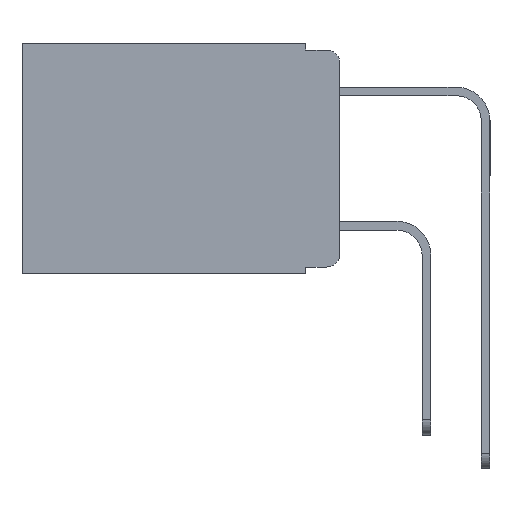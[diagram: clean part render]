
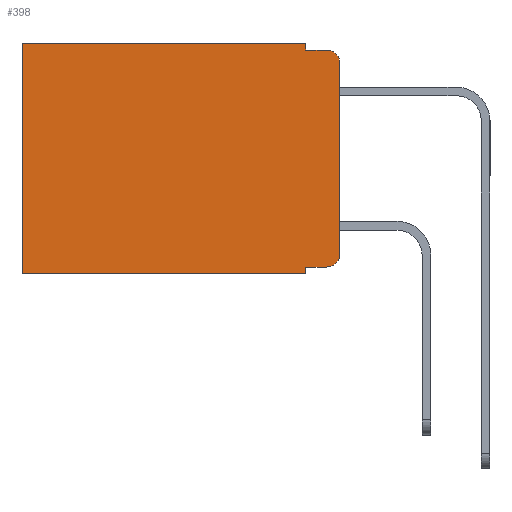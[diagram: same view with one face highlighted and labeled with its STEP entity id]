
A CAD part, left-side view. The second image highlights one B-rep face of the part: STEP entity #398.
In plain terms, the highlighted planar face has unit normal (-1, 0, 0).
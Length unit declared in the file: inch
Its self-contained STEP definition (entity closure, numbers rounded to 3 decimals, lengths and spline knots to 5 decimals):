
#398 = ADVANCED_FACE ( 'NONE', ( #4030 ), #1964, .F. ) ;
#579 = DIRECTION ( 'NONE',  ( 0., 0., -1. ) ) ;
#777 = CARTESIAN_POINT ( 'NONE',  ( 0.298, 0.02, -0.01 ) ) ;
#1148 = ORIENTED_EDGE ( 'NONE', *, *, #8814, .T. ) ;
#1375 = CARTESIAN_POINT ( 'NONE',  ( 0.298, 0.051, 0. ) ) ;
#1418 = LINE ( 'NONE', #10585, #7453 ) ;
#1426 = EDGE_LOOP ( 'NONE', ( #7088, #9582, #7690, #4832, #8796, #1148, #4057, #6673, #2758, #2745 ) ) ;
#1887 = DIRECTION ( 'NONE',  ( 0., 0., -1. ) ) ;
#1944 = DIRECTION ( 'NONE',  ( 1., 0., 0. ) ) ;
#1964 = PLANE ( 'NONE',  #11929 ) ;
#2343 = VERTEX_POINT ( 'NONE', #12642 ) ;
#2522 = CARTESIAN_POINT ( 'NONE',  ( 0.298, 0., -0.313 ) ) ;
#2745 = ORIENTED_EDGE ( 'NONE', *, *, #8131, .T. ) ;
#2758 = ORIENTED_EDGE ( 'NONE', *, *, #8881, .T. ) ;
#3230 = VECTOR ( 'NONE', #5538, 39.37008 ) ;
#3238 = CIRCLE ( 'NONE', #13458, 0.02 ) ;
#3436 = LINE ( 'NONE', #7228, #9574 ) ;
#3459 = CARTESIAN_POINT ( 'NONE',  ( 0.298, 0.02, -0.333 ) ) ;
#3597 = VERTEX_POINT ( 'NONE', #777 ) ;
#4030 = FACE_OUTER_BOUND ( 'NONE', #1426, .T. ) ;
#4057 = ORIENTED_EDGE ( 'NONE', *, *, #8370, .F. ) ;
#4218 = CARTESIAN_POINT ( 'NONE',  ( 0.298, 0.051, 0. ) ) ;
#4225 = LINE ( 'NONE', #8294, #13107 ) ;
#4435 = LINE ( 'NONE', #10112, #10408 ) ;
#4832 = ORIENTED_EDGE ( 'NONE', *, *, #8698, .F. ) ;
#4881 = VERTEX_POINT ( 'NONE', #2522 ) ;
#4936 = VERTEX_POINT ( 'NONE', #1375 ) ;
#5086 = CARTESIAN_POINT ( 'NONE',  ( 0.298, 0.02, -0.313 ) ) ;
#5538 = DIRECTION ( 'NONE',  ( 0., 0., -1. ) ) ;
#6018 = CARTESIAN_POINT ( 'NONE',  ( 0.298, 0.051, -0.333 ) ) ;
#6340 = DIRECTION ( 'NONE',  ( 0., 0., -1. ) ) ;
#6500 = VERTEX_POINT ( 'NONE', #13370 ) ;
#6637 = LINE ( 'NONE', #4218, #3230 ) ;
#6673 = ORIENTED_EDGE ( 'NONE', *, *, #8855, .F. ) ;
#6739 = DIRECTION ( 'NONE',  ( -1., 0., 0. ) ) ;
#6950 = VERTEX_POINT ( 'NONE', #12296 ) ;
#7088 = ORIENTED_EDGE ( 'NONE', *, *, #8621, .F. ) ;
#7228 = CARTESIAN_POINT ( 'NONE',  ( 0.298, 0.051, 0. ) ) ;
#7453 = VECTOR ( 'NONE', #11687, 39.37008 ) ;
#7690 = ORIENTED_EDGE ( 'NONE', *, *, #8696, .F. ) ;
#8131 = EDGE_CURVE ( 'NONE', #8392, #4881, #3238, .T. ) ;
#8294 = CARTESIAN_POINT ( 'NONE',  ( 0.298, 0.473, 0. ) ) ;
#8370 = EDGE_CURVE ( 'NONE', #15028, #2343, #1418, .T. ) ;
#8392 = VERTEX_POINT ( 'NONE', #3459 ) ;
#8451 = DIRECTION ( 'NONE',  ( 0., 0., -1. ) ) ;
#8621 = EDGE_CURVE ( 'NONE', #11386, #4881, #11075, .T. ) ;
#8651 = EDGE_CURVE ( 'NONE', #4936, #12605, #4435, .T. ) ;
#8675 = EDGE_CURVE ( 'NONE', #11386, #3597, #13286, .T. ) ;
#8696 = EDGE_CURVE ( 'NONE', #6500, #3597, #12942, .T. ) ;
#8698 = EDGE_CURVE ( 'NONE', #4936, #6500, #6637, .T. ) ;
#8796 = ORIENTED_EDGE ( 'NONE', *, *, #8651, .T. ) ;
#8814 = EDGE_CURVE ( 'NONE', #12605, #2343, #4225, .T. ) ;
#8848 = CARTESIAN_POINT ( 'NONE',  ( 0.298, 0., -0.03 ) ) ;
#8855 = EDGE_CURVE ( 'NONE', #6950, #15028, #3436, .T. ) ;
#8881 = EDGE_CURVE ( 'NONE', #6950, #8392, #9900, .T. ) ;
#9029 = CARTESIAN_POINT ( 'NONE',  ( 0.298, 0., 0. ) ) ;
#9574 = VECTOR ( 'NONE', #8451, 39.37008 ) ;
#9582 = ORIENTED_EDGE ( 'NONE', *, *, #8675, .T. ) ;
#9745 = VECTOR ( 'NONE', #12364, 39.37008 ) ;
#9900 = LINE ( 'NONE', #6018, #12084 ) ;
#10112 = CARTESIAN_POINT ( 'NONE',  ( 0.298, 0., 0. ) ) ;
#10210 = CARTESIAN_POINT ( 'NONE',  ( 0.298, 0.051, -0.01 ) ) ;
#10408 = VECTOR ( 'NONE', #11188, 39.37008 ) ;
#10585 = CARTESIAN_POINT ( 'NONE',  ( 0.298, 0., -0.343 ) ) ;
#10665 = DIRECTION ( 'NONE',  ( 0., -1., 0. ) ) ;
#11075 = LINE ( 'NONE', #9029, #13933 ) ;
#11188 = DIRECTION ( 'NONE',  ( 0., 1., 0. ) ) ;
#11386 = VERTEX_POINT ( 'NONE', #8848 ) ;
#11687 = DIRECTION ( 'NONE',  ( 0., 1., 0. ) ) ;
#11929 = AXIS2_PLACEMENT_3D ( 'NONE', #13484, #1944, #1887 ) ;
#12084 = VECTOR ( 'NONE', #10665, 39.37008 ) ;
#12296 = CARTESIAN_POINT ( 'NONE',  ( 0.298, 0.051, -0.333 ) ) ;
#12364 = DIRECTION ( 'NONE',  ( 0., -1., 0. ) ) ;
#12605 = VERTEX_POINT ( 'NONE', #15211 ) ;
#12642 = CARTESIAN_POINT ( 'NONE',  ( 0.298, 0.473, -0.343 ) ) ;
#12942 = LINE ( 'NONE', #10210, #9745 ) ;
#13075 = DIRECTION ( 'NONE',  ( -1., 0., 0. ) ) ;
#13107 = VECTOR ( 'NONE', #579, 39.37008 ) ;
#13281 = DIRECTION ( 'NONE',  ( 0., 0., -1. ) ) ;
#13286 = CIRCLE ( 'NONE', #13624, 0.02 ) ;
#13370 = CARTESIAN_POINT ( 'NONE',  ( 0.298, 0.051, -0.01 ) ) ;
#13418 = CARTESIAN_POINT ( 'NONE',  ( 0.298, 0.02, -0.03 ) ) ;
#13458 = AXIS2_PLACEMENT_3D ( 'NONE', #5086, #13075, #6340 ) ;
#13484 = CARTESIAN_POINT ( 'NONE',  ( 0.298, 0., 0. ) ) ;
#13624 = AXIS2_PLACEMENT_3D ( 'NONE', #13418, #6739, #14444 ) ;
#13933 = VECTOR ( 'NONE', #13281, 39.37008 ) ;
#14340 = CARTESIAN_POINT ( 'NONE',  ( 0.298, 0.051, -0.343 ) ) ;
#14444 = DIRECTION ( 'NONE',  ( 0., 0., -1. ) ) ;
#15028 = VERTEX_POINT ( 'NONE', #14340 ) ;
#15211 = CARTESIAN_POINT ( 'NONE',  ( 0.298, 0.473, 0. ) ) ;
